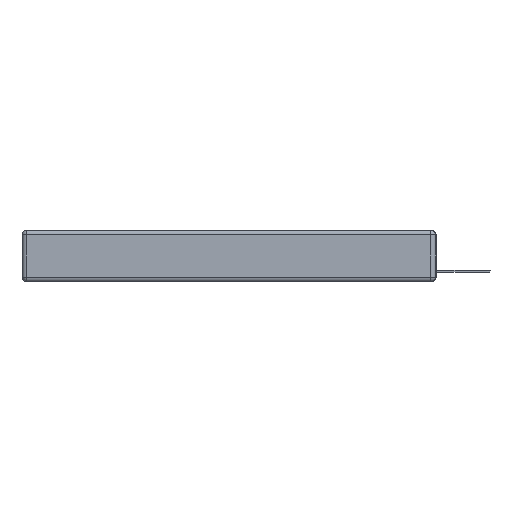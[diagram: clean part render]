
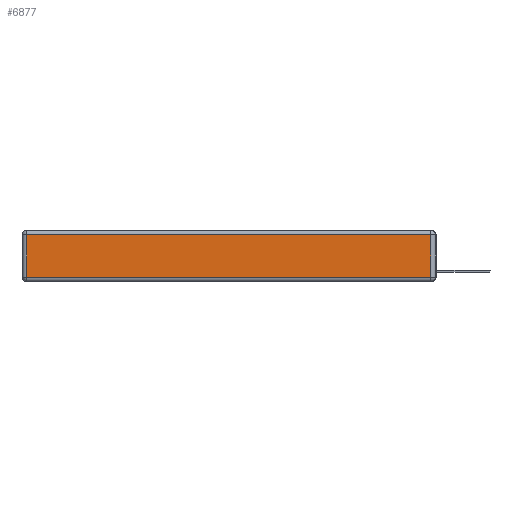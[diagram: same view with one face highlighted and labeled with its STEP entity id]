
A CAD part, left-side view. The second image highlights one B-rep face of the part: STEP entity #6877.
In plain terms, the highlighted planar face has unit normal (-1, 0, 0).
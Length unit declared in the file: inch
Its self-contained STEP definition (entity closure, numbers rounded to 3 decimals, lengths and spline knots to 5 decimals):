
#21 = EDGE_CURVE ( 'NONE', #24424, #11411, #10948, .T. ) ;
#1140 = EDGE_CURVE ( 'NONE', #2701, #24424, #7831, .T. ) ;
#2521 = DIRECTION ( 'NONE',  ( 0., 0., 1. ) ) ;
#2701 = VERTEX_POINT ( 'NONE', #9755 ) ;
#2814 = VECTOR ( 'NONE', #5659, 39.37008 ) ;
#3112 = CARTESIAN_POINT ( 'NONE',  ( 0., 2.75, -0.03 ) ) ;
#5199 = VECTOR ( 'NONE', #24624, 39.37008 ) ;
#5659 = DIRECTION ( 'NONE',  ( 0., 1., 0. ) ) ;
#6877 = ADVANCED_FACE ( 'NONE', ( #20539 ), #19956, .T. ) ;
#7021 = EDGE_LOOP ( 'NONE', ( #7494, #19362, #19048, #20796 ) ) ;
#7127 = CARTESIAN_POINT ( 'NONE',  ( 0., 0., -0.343 ) ) ;
#7494 = ORIENTED_EDGE ( 'NONE', *, *, #21, .T. ) ;
#7831 = LINE ( 'NONE', #14330, #22223 ) ;
#9755 = CARTESIAN_POINT ( 'NONE',  ( 0., 2.72, -0.03 ) ) ;
#10194 = CARTESIAN_POINT ( 'NONE',  ( 0., 0.03, -0.313 ) ) ;
#10453 = VERTEX_POINT ( 'NONE', #12881 ) ;
#10948 = LINE ( 'NONE', #22507, #5199 ) ;
#11037 = EDGE_CURVE ( 'NONE', #11411, #10453, #14854, .T. ) ;
#11411 = VERTEX_POINT ( 'NONE', #10194 ) ;
#11915 = DIRECTION ( 'NONE',  ( 0., 0., -1. ) ) ;
#12812 = CARTESIAN_POINT ( 'NONE',  ( 0., 0.03, -0.343 ) ) ;
#12881 = CARTESIAN_POINT ( 'NONE',  ( 0., 0.03, -0.03 ) ) ;
#14330 = CARTESIAN_POINT ( 'NONE',  ( 0., 2.72, -0.343 ) ) ;
#14854 = LINE ( 'NONE', #12812, #21856 ) ;
#16274 = AXIS2_PLACEMENT_3D ( 'NONE', #7127, #17586, #22105 ) ;
#17463 = EDGE_CURVE ( 'NONE', #10453, #2701, #20601, .T. ) ;
#17496 = CARTESIAN_POINT ( 'NONE',  ( 0., 2.72, -0.313 ) ) ;
#17586 = DIRECTION ( 'NONE',  ( -1., 0., 0. ) ) ;
#19048 = ORIENTED_EDGE ( 'NONE', *, *, #17463, .T. ) ;
#19362 = ORIENTED_EDGE ( 'NONE', *, *, #11037, .T. ) ;
#19956 = PLANE ( 'NONE',  #16274 ) ;
#20539 = FACE_OUTER_BOUND ( 'NONE', #7021, .T. ) ;
#20601 = LINE ( 'NONE', #3112, #2814 ) ;
#20796 = ORIENTED_EDGE ( 'NONE', *, *, #1140, .T. ) ;
#21856 = VECTOR ( 'NONE', #2521, 39.37008 ) ;
#22105 = DIRECTION ( 'NONE',  ( 0., 0., 1. ) ) ;
#22223 = VECTOR ( 'NONE', #11915, 39.37008 ) ;
#22507 = CARTESIAN_POINT ( 'NONE',  ( 0., 0., -0.313 ) ) ;
#24424 = VERTEX_POINT ( 'NONE', #17496 ) ;
#24624 = DIRECTION ( 'NONE',  ( 0., -1., 0. ) ) ;
